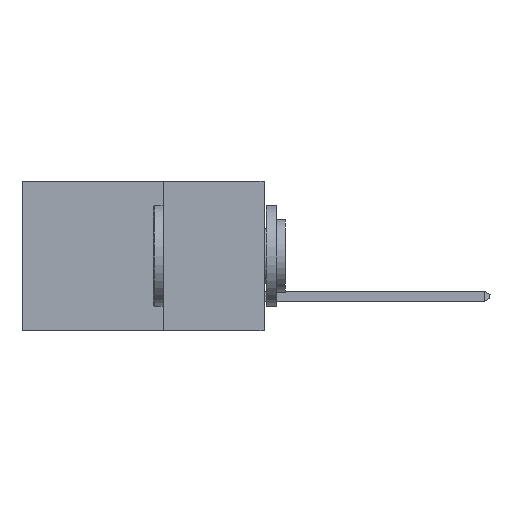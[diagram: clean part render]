
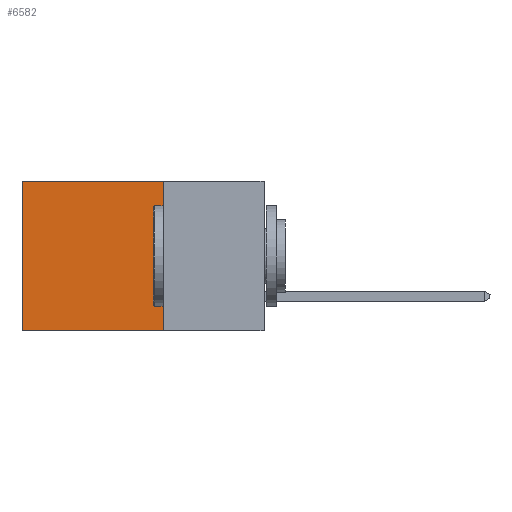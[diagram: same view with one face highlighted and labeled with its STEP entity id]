
A CAD part, left-side view. The second image highlights one B-rep face of the part: STEP entity #6582.
In plain terms, the highlighted planar face has unit normal (-1, 0, 0).
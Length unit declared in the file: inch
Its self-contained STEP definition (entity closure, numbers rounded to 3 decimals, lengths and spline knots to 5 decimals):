
#193 = VERTEX_POINT ( 'NONE', #1728 ) ;
#884 = DIRECTION ( 'NONE',  ( 0., 0., -1. ) ) ;
#976 = LINE ( 'NONE', #5242, #2379 ) ;
#1488 = AXIS2_PLACEMENT_3D ( 'NONE', #13625, #9239, #884 ) ;
#1728 = CARTESIAN_POINT ( 'NONE',  ( 0.2615, 0.6, 0. ) ) ;
#2231 = CARTESIAN_POINT ( 'NONE',  ( 0.2615, 0.25, -0.37 ) ) ;
#2379 = VECTOR ( 'NONE', #10367, 39.37008 ) ;
#3012 = CARTESIAN_POINT ( 'NONE',  ( 0.2615, 0.25, 0. ) ) ;
#3382 = ORIENTED_EDGE ( 'NONE', *, *, #4784, .T. ) ;
#3809 = VECTOR ( 'NONE', #10399, 39.37008 ) ;
#4067 = DIRECTION ( 'NONE',  ( 0., 1., 0. ) ) ;
#4739 = ORIENTED_EDGE ( 'NONE', *, *, #4828, .T. ) ;
#4784 = EDGE_CURVE ( 'NONE', #6488, #193, #8259, .T. ) ;
#4828 = EDGE_CURVE ( 'NONE', #193, #12896, #976, .T. ) ;
#5242 = CARTESIAN_POINT ( 'NONE',  ( 0.2615, 0.6, -0.37 ) ) ;
#6169 = VECTOR ( 'NONE', #4067, 39.37008 ) ;
#6189 = ORIENTED_EDGE ( 'NONE', *, *, #7929, .F. ) ;
#6260 = LINE ( 'NONE', #7110, #3809 ) ;
#6382 = ORIENTED_EDGE ( 'NONE', *, *, #9706, .F. ) ;
#6488 = VERTEX_POINT ( 'NONE', #11599 ) ;
#6582 = ADVANCED_FACE ( 'NONE', ( #7128 ), #10622, .F. ) ;
#7110 = CARTESIAN_POINT ( 'NONE',  ( 0.2615, 0.25, -0.37 ) ) ;
#7128 = FACE_OUTER_BOUND ( 'NONE', #9318, .T. ) ;
#7468 = DIRECTION ( 'NONE',  ( 0., 0., -1. ) ) ;
#7701 = CARTESIAN_POINT ( 'NONE',  ( 0.2615, 0.25, -0.37 ) ) ;
#7717 = CARTESIAN_POINT ( 'NONE',  ( 0.2615, 0.6, -0.37 ) ) ;
#7929 = EDGE_CURVE ( 'NONE', #6488, #9238, #12990, .T. ) ;
#8259 = LINE ( 'NONE', #3012, #6169 ) ;
#9238 = VERTEX_POINT ( 'NONE', #7701 ) ;
#9239 = DIRECTION ( 'NONE',  ( 1., 0., 0. ) ) ;
#9318 = EDGE_LOOP ( 'NONE', ( #4739, #6382, #6189, #3382 ) ) ;
#9706 = EDGE_CURVE ( 'NONE', #9238, #12896, #6260, .T. ) ;
#10367 = DIRECTION ( 'NONE',  ( 0., 0., -1. ) ) ;
#10399 = DIRECTION ( 'NONE',  ( 0., 1., 0. ) ) ;
#10453 = VECTOR ( 'NONE', #7468, 39.37008 ) ;
#10622 = PLANE ( 'NONE',  #1488 ) ;
#11599 = CARTESIAN_POINT ( 'NONE',  ( 0.2615, 0.25, 0. ) ) ;
#12896 = VERTEX_POINT ( 'NONE', #7717 ) ;
#12990 = LINE ( 'NONE', #2231, #10453 ) ;
#13625 = CARTESIAN_POINT ( 'NONE',  ( 0.2615, 0.25, -0.37 ) ) ;
